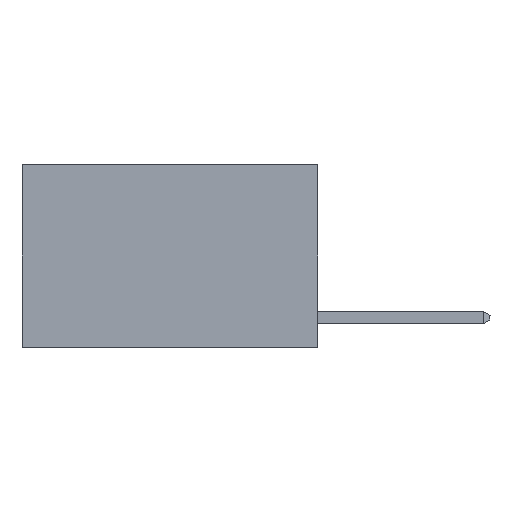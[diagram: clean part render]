
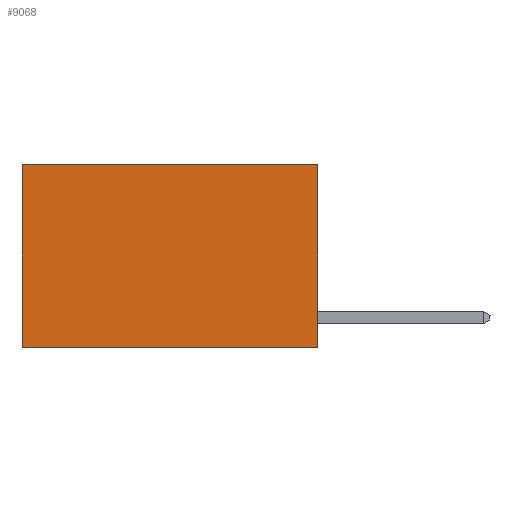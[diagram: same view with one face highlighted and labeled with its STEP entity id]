
A CAD part, left-side view. The second image highlights one B-rep face of the part: STEP entity #9068.
In plain terms, the highlighted planar face has unit normal (-1, 0, 0).
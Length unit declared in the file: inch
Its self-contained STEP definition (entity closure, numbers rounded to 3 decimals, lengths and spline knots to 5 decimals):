
#181 = CARTESIAN_POINT ( 'NONE',  ( 0.2625, 0., -0.37 ) ) ;
#634 = VECTOR ( 'NONE', #11045, 39.37008 ) ;
#1153 = DIRECTION ( 'NONE',  ( 0., 0., -1. ) ) ;
#1318 = LINE ( 'NONE', #19597, #4494 ) ;
#2380 = DIRECTION ( 'NONE',  ( 0., 1., 0. ) ) ;
#2988 = EDGE_CURVE ( 'NONE', #15589, #9250, #1318, .T. ) ;
#3849 = VECTOR ( 'NONE', #2380, 39.37008 ) ;
#4029 = VECTOR ( 'NONE', #15804, 39.37008 ) ;
#4099 = EDGE_LOOP ( 'NONE', ( #12551, #14682, #5116, #10253 ) ) ;
#4494 = VECTOR ( 'NONE', #1153, 39.37008 ) ;
#4541 = EDGE_CURVE ( 'NONE', #9250, #11413, #12503, .T. ) ;
#5116 = ORIENTED_EDGE ( 'NONE', *, *, #2988, .F. ) ;
#5372 = FACE_OUTER_BOUND ( 'NONE', #4099, .T. ) ;
#5459 = CARTESIAN_POINT ( 'NONE',  ( 0.2625, 0., 0. ) ) ;
#7629 = DIRECTION ( 'NONE',  ( 1., 0., 0. ) ) ;
#9068 = ADVANCED_FACE ( 'NONE', ( #5372 ), #13713, .F. ) ;
#9250 = VERTEX_POINT ( 'NONE', #14232 ) ;
#10253 = ORIENTED_EDGE ( 'NONE', *, *, #15747, .T. ) ;
#10359 = VERTEX_POINT ( 'NONE', #10781 ) ;
#10781 = CARTESIAN_POINT ( 'NONE',  ( 0.2625, 0.6, 0. ) ) ;
#11045 = DIRECTION ( 'NONE',  ( 0., 1., 0. ) ) ;
#11229 = CARTESIAN_POINT ( 'NONE',  ( 0.2625, 0., 0. ) ) ;
#11256 = LINE ( 'NONE', #12747, #4029 ) ;
#11413 = VERTEX_POINT ( 'NONE', #17721 ) ;
#12503 = LINE ( 'NONE', #181, #634 ) ;
#12551 = ORIENTED_EDGE ( 'NONE', *, *, #17601, .T. ) ;
#12747 = CARTESIAN_POINT ( 'NONE',  ( 0.2625, 0.6, 0. ) ) ;
#13088 = AXIS2_PLACEMENT_3D ( 'NONE', #18269, #7629, #18334 ) ;
#13713 = PLANE ( 'NONE',  #13088 ) ;
#14232 = CARTESIAN_POINT ( 'NONE',  ( 0.2625, 0., -0.37 ) ) ;
#14682 = ORIENTED_EDGE ( 'NONE', *, *, #4541, .F. ) ;
#15589 = VERTEX_POINT ( 'NONE', #11229 ) ;
#15747 = EDGE_CURVE ( 'NONE', #15589, #10359, #19689, .T. ) ;
#15804 = DIRECTION ( 'NONE',  ( 0., 0., -1. ) ) ;
#17601 = EDGE_CURVE ( 'NONE', #10359, #11413, #11256, .T. ) ;
#17721 = CARTESIAN_POINT ( 'NONE',  ( 0.2625, 0.6, -0.37 ) ) ;
#18269 = CARTESIAN_POINT ( 'NONE',  ( 0.2625, 0., 0. ) ) ;
#18334 = DIRECTION ( 'NONE',  ( 0., 0., -1. ) ) ;
#19597 = CARTESIAN_POINT ( 'NONE',  ( 0.2625, 0., 0. ) ) ;
#19689 = LINE ( 'NONE', #5459, #3849 ) ;
